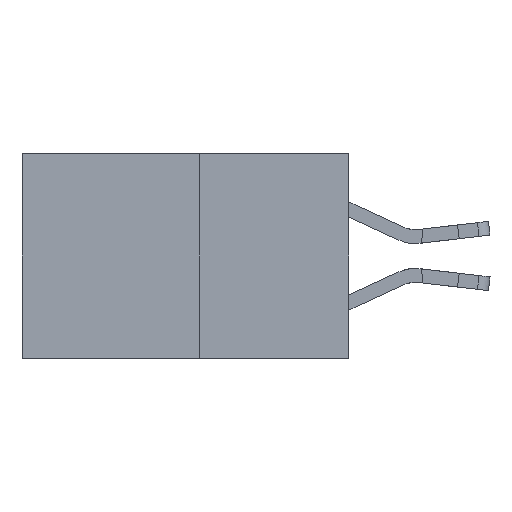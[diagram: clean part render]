
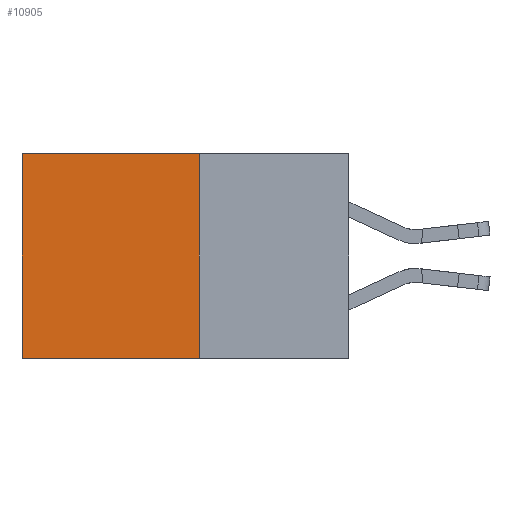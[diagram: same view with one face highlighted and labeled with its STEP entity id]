
A CAD part, left-side view. The second image highlights one B-rep face of the part: STEP entity #10905.
In plain terms, the highlighted planar face has unit normal (-1, 0, 0).
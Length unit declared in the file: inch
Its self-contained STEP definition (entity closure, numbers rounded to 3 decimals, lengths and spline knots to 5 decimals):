
#168 = DIRECTION ( 'NONE',  ( 0., 0., -1. ) ) ;
#299 = LINE ( 'NONE', #14156, #11767 ) ;
#1611 = ORIENTED_EDGE ( 'NONE', *, *, #17050, .F. ) ;
#1932 = VERTEX_POINT ( 'NONE', #11714 ) ;
#3440 = VECTOR ( 'NONE', #15654, 39.37008 ) ;
#3576 = CARTESIAN_POINT ( 'NONE',  ( 0.277, 0.27, -0.37 ) ) ;
#3871 = ORIENTED_EDGE ( 'NONE', *, *, #19605, .T. ) ;
#4465 = ORIENTED_EDGE ( 'NONE', *, *, #17982, .T. ) ;
#5639 = CARTESIAN_POINT ( 'NONE',  ( 0.277, 0.59, 0. ) ) ;
#5895 = EDGE_CURVE ( 'NONE', #19421, #18685, #10496, .T. ) ;
#6220 = FACE_OUTER_BOUND ( 'NONE', #7100, .T. ) ;
#6293 = LINE ( 'NONE', #11737, #16751 ) ;
#7091 = DIRECTION ( 'NONE',  ( 0., 1., 0. ) ) ;
#7100 = EDGE_LOOP ( 'NONE', ( #4465, #14979, #1611, #3871 ) ) ;
#7941 = PLANE ( 'NONE',  #12434 ) ;
#8319 = DIRECTION ( 'NONE',  ( 0., 0., -1. ) ) ;
#9504 = DIRECTION ( 'NONE',  ( 1., 0., 0. ) ) ;
#10496 = LINE ( 'NONE', #12274, #14163 ) ;
#10905 = ADVANCED_FACE ( 'NONE', ( #6220 ), #7941, .F. ) ;
#10962 = CARTESIAN_POINT ( 'NONE',  ( 0.277, 0.59, -0.37 ) ) ;
#11714 = CARTESIAN_POINT ( 'NONE',  ( 0.277, 0.27, 0. ) ) ;
#11737 = CARTESIAN_POINT ( 'NONE',  ( 0.277, 0.27, 0. ) ) ;
#11767 = VECTOR ( 'NONE', #8319, 39.37008 ) ;
#12274 = CARTESIAN_POINT ( 'NONE',  ( 0.277, 0.27, -0.37 ) ) ;
#12434 = AXIS2_PLACEMENT_3D ( 'NONE', #18763, #9504, #168 ) ;
#14156 = CARTESIAN_POINT ( 'NONE',  ( 0.277, 0.27, -0.37 ) ) ;
#14163 = VECTOR ( 'NONE', #16140, 39.37008 ) ;
#14644 = VERTEX_POINT ( 'NONE', #5639 ) ;
#14979 = ORIENTED_EDGE ( 'NONE', *, *, #5895, .F. ) ;
#15341 = LINE ( 'NONE', #10962, #3440 ) ;
#15654 = DIRECTION ( 'NONE',  ( 0., 0., -1. ) ) ;
#16140 = DIRECTION ( 'NONE',  ( 0., 1., 0. ) ) ;
#16751 = VECTOR ( 'NONE', #7091, 39.37008 ) ;
#17050 = EDGE_CURVE ( 'NONE', #1932, #19421, #299, .T. ) ;
#17982 = EDGE_CURVE ( 'NONE', #14644, #18685, #15341, .T. ) ;
#18685 = VERTEX_POINT ( 'NONE', #18699 ) ;
#18699 = CARTESIAN_POINT ( 'NONE',  ( 0.277, 0.59, -0.37 ) ) ;
#18763 = CARTESIAN_POINT ( 'NONE',  ( 0.277, 0.27, -0.37 ) ) ;
#19421 = VERTEX_POINT ( 'NONE', #3576 ) ;
#19605 = EDGE_CURVE ( 'NONE', #1932, #14644, #6293, .T. ) ;
